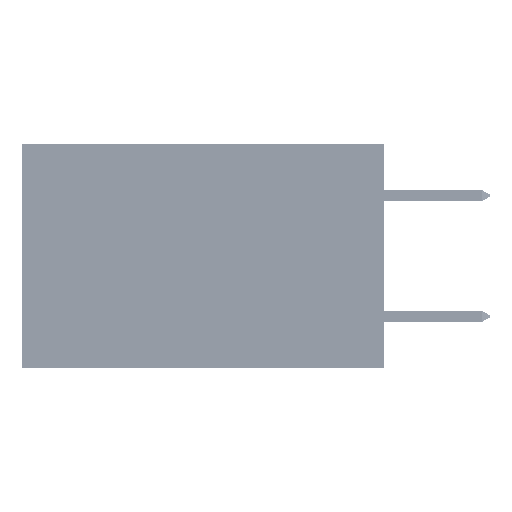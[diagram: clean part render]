
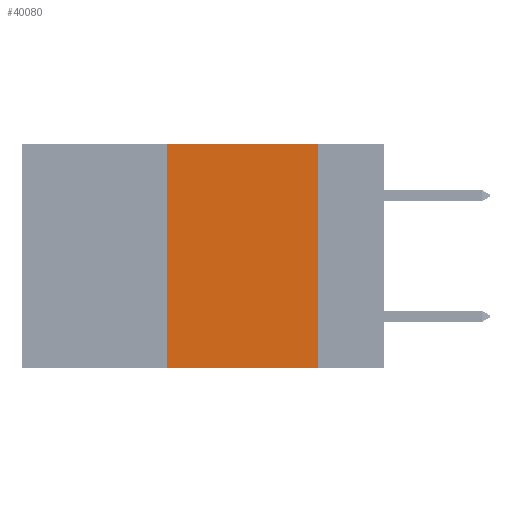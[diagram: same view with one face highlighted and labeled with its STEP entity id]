
A CAD part, left-side view. The second image highlights one B-rep face of the part: STEP entity #40080.
In plain terms, the highlighted planar face has unit normal (-1, 0, 0).
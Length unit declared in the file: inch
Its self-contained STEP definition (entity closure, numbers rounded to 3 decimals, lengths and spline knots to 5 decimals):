
#1494 = DIRECTION ( 'NONE',  ( 0., 0., -1. ) ) ;
#1708 = VERTEX_POINT ( 'NONE', #17668 ) ;
#3831 = ORIENTED_EDGE ( 'NONE', *, *, #28104, .F. ) ;
#4197 = LINE ( 'NONE', #41788, #34076 ) ;
#5479 = CARTESIAN_POINT ( 'NONE',  ( 0., 0.6, -0.37 ) ) ;
#8218 = ORIENTED_EDGE ( 'NONE', *, *, #48303, .T. ) ;
#8349 = LINE ( 'NONE', #20825, #40154 ) ;
#11306 = AXIS2_PLACEMENT_3D ( 'NONE', #29734, #25807, #1494 ) ;
#13724 = CARTESIAN_POINT ( 'NONE',  ( 0., 0.6, 0. ) ) ;
#14063 = VERTEX_POINT ( 'NONE', #16546 ) ;
#14629 = FACE_OUTER_BOUND ( 'NONE', #24273, .T. ) ;
#16546 = CARTESIAN_POINT ( 'NONE',  ( 0., 0.11, 0. ) ) ;
#17668 = CARTESIAN_POINT ( 'NONE',  ( 0., 0.36, 0. ) ) ;
#19200 = VECTOR ( 'NONE', #33988, 39.37008 ) ;
#20825 = CARTESIAN_POINT ( 'NONE',  ( 0., 0.11, 0. ) ) ;
#24273 = EDGE_LOOP ( 'NONE', ( #46222, #45800, #3831, #8218 ) ) ;
#25807 = DIRECTION ( 'NONE',  ( 1., 0., 0. ) ) ;
#27335 = CARTESIAN_POINT ( 'NONE',  ( 0., 0.11, -0.37 ) ) ;
#28104 = EDGE_CURVE ( 'NONE', #28489, #1708, #4197, .T. ) ;
#28489 = VERTEX_POINT ( 'NONE', #44038 ) ;
#29734 = CARTESIAN_POINT ( 'NONE',  ( 0., 0.6, 0. ) ) ;
#32987 = VERTEX_POINT ( 'NONE', #27335 ) ;
#33335 = EDGE_CURVE ( 'NONE', #1708, #14063, #35721, .T. ) ;
#33988 = DIRECTION ( 'NONE',  ( 0., -1., 0. ) ) ;
#34076 = VECTOR ( 'NONE', #46180, 39.37008 ) ;
#34172 = PLANE ( 'NONE',  #11306 ) ;
#35721 = LINE ( 'NONE', #13724, #19200 ) ;
#38404 = LINE ( 'NONE', #5479, #50442 ) ;
#40080 = ADVANCED_FACE ( 'NONE', ( #14629 ), #34172, .F. ) ;
#40154 = VECTOR ( 'NONE', #49224, 39.37008 ) ;
#41788 = CARTESIAN_POINT ( 'NONE',  ( 0., 0.36, 0. ) ) ;
#44038 = CARTESIAN_POINT ( 'NONE',  ( 0., 0.36, -0.37 ) ) ;
#45800 = ORIENTED_EDGE ( 'NONE', *, *, #33335, .F. ) ;
#46180 = DIRECTION ( 'NONE',  ( 0., 0., 1. ) ) ;
#46222 = ORIENTED_EDGE ( 'NONE', *, *, #49562, .F. ) ;
#48303 = EDGE_CURVE ( 'NONE', #28489, #32987, #38404, .T. ) ;
#49224 = DIRECTION ( 'NONE',  ( 0., 0., -1. ) ) ;
#49562 = EDGE_CURVE ( 'NONE', #14063, #32987, #8349, .T. ) ;
#49881 = DIRECTION ( 'NONE',  ( 0., -1., 0. ) ) ;
#50442 = VECTOR ( 'NONE', #49881, 39.37008 ) ;
